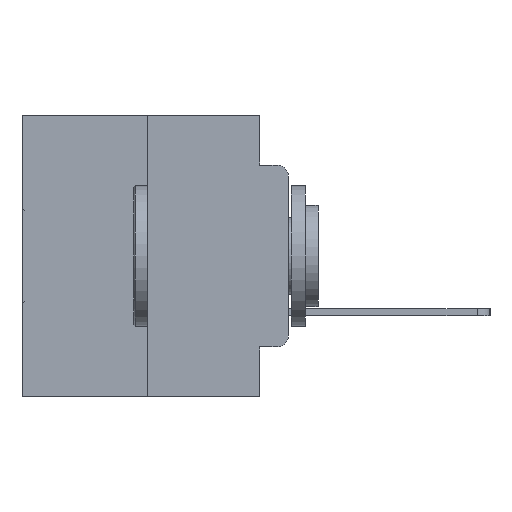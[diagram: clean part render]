
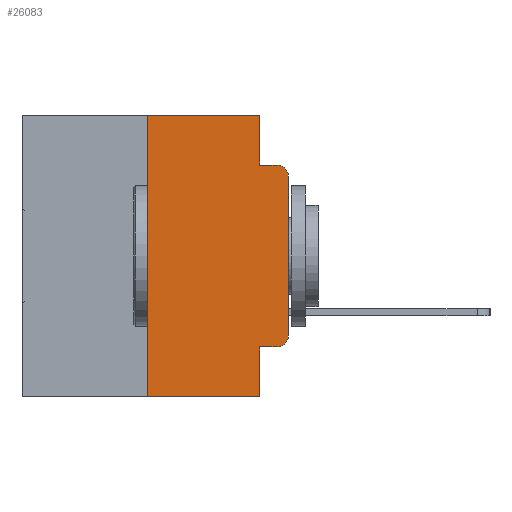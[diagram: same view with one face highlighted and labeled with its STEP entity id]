
A CAD part, left-side view. The second image highlights one B-rep face of the part: STEP entity #26083.
In plain terms, the highlighted planar face has unit normal (-1, 0, 0).
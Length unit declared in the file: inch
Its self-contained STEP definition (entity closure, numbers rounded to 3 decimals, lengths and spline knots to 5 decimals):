
#480 = EDGE_CURVE ( 'NONE', #2062, #24380, #3981, .T. ) ;
#886 = PLANE ( 'NONE',  #22155 ) ;
#938 = LINE ( 'NONE', #1191, #13229 ) ;
#1121 = CARTESIAN_POINT ( 'NONE',  ( 0., 0.25, -0.5 ) ) ;
#1191 = CARTESIAN_POINT ( 'NONE',  ( 0., 0.051, -0.4115 ) ) ;
#1334 = ORIENTED_EDGE ( 'NONE', *, *, #3972, .F. ) ;
#1505 = LINE ( 'NONE', #25057, #7509 ) ;
#1536 = LINE ( 'NONE', #7694, #8285 ) ;
#1776 = CARTESIAN_POINT ( 'NONE',  ( 0., 0.051, -0.4115 ) ) ;
#2062 = VERTEX_POINT ( 'NONE', #1121 ) ;
#2224 = VECTOR ( 'NONE', #27793, 39.37008 ) ;
#2264 = EDGE_CURVE ( 'NONE', #26246, #18380, #1536, .T. ) ;
#2713 = EDGE_CURVE ( 'NONE', #2062, #4123, #1505, .T. ) ;
#2873 = CIRCLE ( 'NONE', #20685, 0.02 ) ;
#3521 = DIRECTION ( 'NONE',  ( 0., 0., -1. ) ) ;
#3784 = ORIENTED_EDGE ( 'NONE', *, *, #2713, .T. ) ;
#3972 = EDGE_CURVE ( 'NONE', #18380, #19469, #5815, .T. ) ;
#3981 = LINE ( 'NONE', #11304, #16621 ) ;
#4123 = VERTEX_POINT ( 'NONE', #27900 ) ;
#5014 = CARTESIAN_POINT ( 'NONE',  ( 0., 0.051, 0. ) ) ;
#5646 = CARTESIAN_POINT ( 'NONE',  ( 0., 0.473, 0. ) ) ;
#5815 = LINE ( 'NONE', #27312, #23858 ) ;
#5864 = VERTEX_POINT ( 'NONE', #11870 ) ;
#7343 = EDGE_CURVE ( 'NONE', #5864, #19469, #11309, .T. ) ;
#7509 = VECTOR ( 'NONE', #28345, 39.37008 ) ;
#7694 = CARTESIAN_POINT ( 'NONE',  ( 0., 0.051, 0. ) ) ;
#8092 = ORIENTED_EDGE ( 'NONE', *, *, #2264, .F. ) ;
#8285 = VECTOR ( 'NONE', #25530, 39.37008 ) ;
#8609 = EDGE_CURVE ( 'NONE', #24380, #26246, #16852, .T. ) ;
#8879 = LINE ( 'NONE', #9145, #2224 ) ;
#8962 = EDGE_CURVE ( 'NONE', #26859, #5864, #8879, .T. ) ;
#9145 = CARTESIAN_POINT ( 'NONE',  ( 0., 0., 0. ) ) ;
#9584 = ORIENTED_EDGE ( 'NONE', *, *, #8609, .F. ) ;
#10773 = VECTOR ( 'NONE', #15145, 39.37008 ) ;
#10824 = DIRECTION ( 'NONE',  ( -1., 0., 0. ) ) ;
#11076 = ORIENTED_EDGE ( 'NONE', *, *, #28311, .F. ) ;
#11304 = CARTESIAN_POINT ( 'NONE',  ( 0., 0.25, 0. ) ) ;
#11309 = CIRCLE ( 'NONE', #26814, 0.02 ) ;
#11419 = ORIENTED_EDGE ( 'NONE', *, *, #8962, .T. ) ;
#11535 = VERTEX_POINT ( 'NONE', #1776 ) ;
#11596 = CARTESIAN_POINT ( 'NONE',  ( 0., 0., -0.3915 ) ) ;
#11870 = CARTESIAN_POINT ( 'NONE',  ( 0., 0., -0.1085 ) ) ;
#12149 = ORIENTED_EDGE ( 'NONE', *, *, #7343, .T. ) ;
#13207 = DIRECTION ( 'NONE',  ( -1., 0., 0. ) ) ;
#13229 = VECTOR ( 'NONE', #22628, 39.37008 ) ;
#13343 = DIRECTION ( 'NONE',  ( 0., -1., 0. ) ) ;
#13810 = CARTESIAN_POINT ( 'NONE',  ( 0., 0.051, 0. ) ) ;
#13853 = CARTESIAN_POINT ( 'NONE',  ( 0., 0.02, -0.0885 ) ) ;
#15040 = FACE_OUTER_BOUND ( 'NONE', #21203, .T. ) ;
#15145 = DIRECTION ( 'NONE',  ( 0., -1., 0. ) ) ;
#15415 = CARTESIAN_POINT ( 'NONE',  ( 0., 0.473, 0. ) ) ;
#16621 = VECTOR ( 'NONE', #27972, 39.37008 ) ;
#16852 = LINE ( 'NONE', #5646, #10773 ) ;
#17148 = ORIENTED_EDGE ( 'NONE', *, *, #26733, .T. ) ;
#17749 = DIRECTION ( 'NONE',  ( 1., 0., 0. ) ) ;
#18380 = VERTEX_POINT ( 'NONE', #24282 ) ;
#18809 = CARTESIAN_POINT ( 'NONE',  ( 0., 0.02, -0.4115 ) ) ;
#19469 = VERTEX_POINT ( 'NONE', #13853 ) ;
#20685 = AXIS2_PLACEMENT_3D ( 'NONE', #27176, #13207, #26273 ) ;
#21203 = EDGE_LOOP ( 'NONE', ( #11419, #12149, #1334, #8092, #9584, #21912, #3784, #11076, #17148, #24876 ) ) ;
#21516 = DIRECTION ( 'NONE',  ( 0., 0., -1. ) ) ;
#21912 = ORIENTED_EDGE ( 'NONE', *, *, #480, .F. ) ;
#21977 = EDGE_CURVE ( 'NONE', #28662, #26859, #2873, .T. ) ;
#22155 = AXIS2_PLACEMENT_3D ( 'NONE', #15415, #17749, #3521 ) ;
#22628 = DIRECTION ( 'NONE',  ( 0., -1., 0. ) ) ;
#23858 = VECTOR ( 'NONE', #13343, 39.37008 ) ;
#24282 = CARTESIAN_POINT ( 'NONE',  ( 0., 0.051, -0.0885 ) ) ;
#24380 = VERTEX_POINT ( 'NONE', #25088 ) ;
#24713 = CARTESIAN_POINT ( 'NONE',  ( 0., 0.02, -0.1085 ) ) ;
#24876 = ORIENTED_EDGE ( 'NONE', *, *, #21977, .T. ) ;
#25057 = CARTESIAN_POINT ( 'NONE',  ( 0., 0.473, -0.5 ) ) ;
#25088 = CARTESIAN_POINT ( 'NONE',  ( 0., 0.25, 0. ) ) ;
#25530 = DIRECTION ( 'NONE',  ( 0., 0., -1. ) ) ;
#26083 = ADVANCED_FACE ( 'NONE', ( #15040 ), #886, .F. ) ;
#26246 = VERTEX_POINT ( 'NONE', #13810 ) ;
#26273 = DIRECTION ( 'NONE',  ( 0., 0., -1. ) ) ;
#26589 = VECTOR ( 'NONE', #21516, 39.37008 ) ;
#26733 = EDGE_CURVE ( 'NONE', #11535, #28662, #938, .T. ) ;
#26814 = AXIS2_PLACEMENT_3D ( 'NONE', #24713, #10824, #27091 ) ;
#26859 = VERTEX_POINT ( 'NONE', #11596 ) ;
#27091 = DIRECTION ( 'NONE',  ( 0., 0., -1. ) ) ;
#27176 = CARTESIAN_POINT ( 'NONE',  ( 0., 0.02, -0.3915 ) ) ;
#27312 = CARTESIAN_POINT ( 'NONE',  ( 0., 0.051, -0.0885 ) ) ;
#27320 = LINE ( 'NONE', #5014, #26589 ) ;
#27793 = DIRECTION ( 'NONE',  ( 0., 0., 1. ) ) ;
#27900 = CARTESIAN_POINT ( 'NONE',  ( 0., 0.051, -0.5 ) ) ;
#27972 = DIRECTION ( 'NONE',  ( 0., 0., 1. ) ) ;
#28311 = EDGE_CURVE ( 'NONE', #11535, #4123, #27320, .T. ) ;
#28345 = DIRECTION ( 'NONE',  ( 0., -1., 0. ) ) ;
#28662 = VERTEX_POINT ( 'NONE', #18809 ) ;
